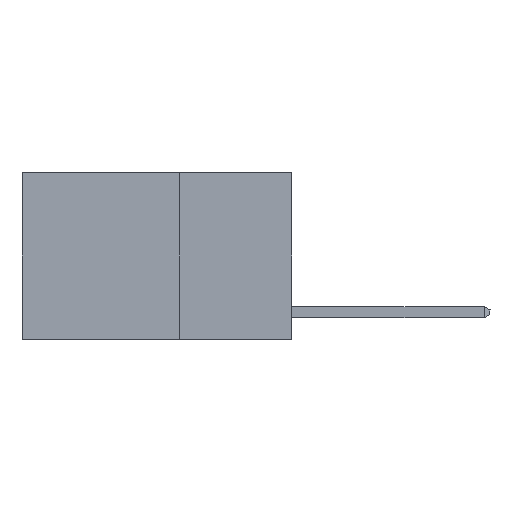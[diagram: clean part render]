
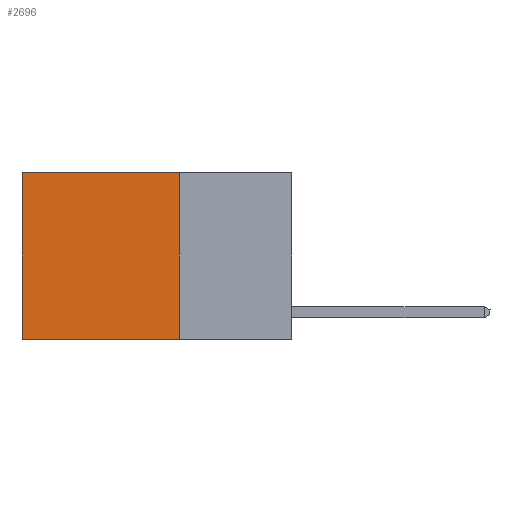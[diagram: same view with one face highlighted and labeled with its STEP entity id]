
A CAD part, left-side view. The second image highlights one B-rep face of the part: STEP entity #2696.
In plain terms, the highlighted planar face has unit normal (-1, 0, 0).
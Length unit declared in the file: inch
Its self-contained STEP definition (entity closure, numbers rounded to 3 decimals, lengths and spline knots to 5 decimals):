
#1346 = EDGE_CURVE ( 'NONE', #4319, #5679, #3913, .T. ) ;
#2064 = VECTOR ( 'NONE', #2917, 39.37008 ) ;
#2120 = ORIENTED_EDGE ( 'NONE', *, *, #10936, .T. ) ;
#2384 = VECTOR ( 'NONE', #3424, 39.37008 ) ;
#2696 = ADVANCED_FACE ( 'NONE', ( #3202 ), #7706, .F. ) ;
#2917 = DIRECTION ( 'NONE',  ( 0., 0., -1. ) ) ;
#2965 = DIRECTION ( 'NONE',  ( 0., 1., 0. ) ) ;
#3202 = FACE_OUTER_BOUND ( 'NONE', #11426, .T. ) ;
#3222 = CARTESIAN_POINT ( 'NONE',  ( 0.2625, 0.25, -0.37 ) ) ;
#3377 = DIRECTION ( 'NONE',  ( 1., 0., 0. ) ) ;
#3424 = DIRECTION ( 'NONE',  ( 0., 0., -1. ) ) ;
#3493 = CARTESIAN_POINT ( 'NONE',  ( 0.2625, 0.6, -0.37 ) ) ;
#3913 = LINE ( 'NONE', #7693, #11570 ) ;
#4075 = ORIENTED_EDGE ( 'NONE', *, *, #11761, .F. ) ;
#4319 = VERTEX_POINT ( 'NONE', #12820 ) ;
#4419 = VERTEX_POINT ( 'NONE', #3222 ) ;
#4524 = CARTESIAN_POINT ( 'NONE',  ( 0.2625, 0.25, 0. ) ) ;
#5362 = ORIENTED_EDGE ( 'NONE', *, *, #1346, .T. ) ;
#5679 = VERTEX_POINT ( 'NONE', #11796 ) ;
#6717 = VERTEX_POINT ( 'NONE', #3493 ) ;
#7418 = ORIENTED_EDGE ( 'NONE', *, *, #9147, .F. ) ;
#7693 = CARTESIAN_POINT ( 'NONE',  ( 0.2625, 0.25, 0. ) ) ;
#7706 = PLANE ( 'NONE',  #12311 ) ;
#8399 = CARTESIAN_POINT ( 'NONE',  ( 0.2625, 0.25, -0.37 ) ) ;
#8770 = DIRECTION ( 'NONE',  ( 0., 1., 0. ) ) ;
#9147 = EDGE_CURVE ( 'NONE', #4419, #6717, #9632, .T. ) ;
#9632 = LINE ( 'NONE', #8399, #13676 ) ;
#9906 = CARTESIAN_POINT ( 'NONE',  ( 0.2625, 0.25, 0. ) ) ;
#10936 = EDGE_CURVE ( 'NONE', #5679, #6717, #13951, .T. ) ;
#10996 = DIRECTION ( 'NONE',  ( 0., 0., -1. ) ) ;
#11426 = EDGE_LOOP ( 'NONE', ( #2120, #7418, #4075, #5362 ) ) ;
#11570 = VECTOR ( 'NONE', #8770, 39.37008 ) ;
#11761 = EDGE_CURVE ( 'NONE', #4319, #4419, #13917, .T. ) ;
#11796 = CARTESIAN_POINT ( 'NONE',  ( 0.2625, 0.6, 0. ) ) ;
#12311 = AXIS2_PLACEMENT_3D ( 'NONE', #9906, #3377, #10996 ) ;
#12707 = CARTESIAN_POINT ( 'NONE',  ( 0.2625, 0.6, 0. ) ) ;
#12820 = CARTESIAN_POINT ( 'NONE',  ( 0.2625, 0.25, 0. ) ) ;
#13676 = VECTOR ( 'NONE', #2965, 39.37008 ) ;
#13917 = LINE ( 'NONE', #4524, #2384 ) ;
#13951 = LINE ( 'NONE', #12707, #2064 ) ;
